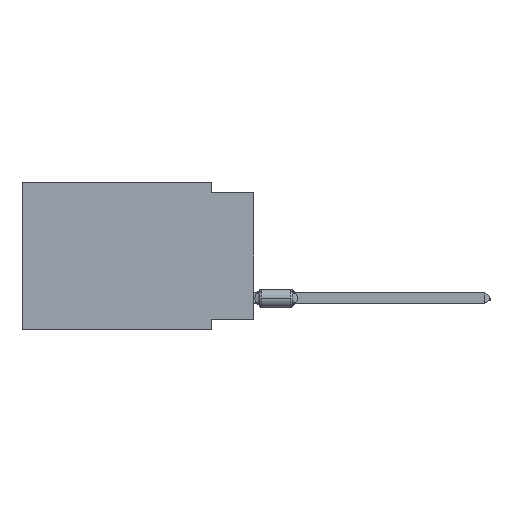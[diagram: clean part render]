
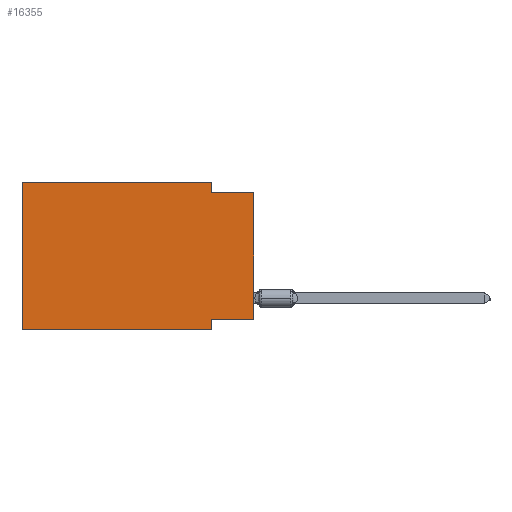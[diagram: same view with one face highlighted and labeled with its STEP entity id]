
A CAD part, left-side view. The second image highlights one B-rep face of the part: STEP entity #16355.
In plain terms, the highlighted planar face has unit normal (-1, 0, 0).
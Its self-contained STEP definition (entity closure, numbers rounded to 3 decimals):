
#432 = CARTESIAN_POINT ( 'NONE',  ( 0., 2.54, 0. ) ) ;
#1191 = EDGE_LOOP ( 'NONE', ( #4856, #4964, #36572, #7061, #2032, #25791, #12695, #21162 ) ) ;
#1422 = VERTEX_POINT ( 'NONE', #13191 ) ;
#2032 = ORIENTED_EDGE ( 'NONE', *, *, #30487, .F. ) ;
#3609 = VERTEX_POINT ( 'NONE', #37012 ) ;
#4856 = ORIENTED_EDGE ( 'NONE', *, *, #19941, .T. ) ;
#4964 = ORIENTED_EDGE ( 'NONE', *, *, #16062, .F. ) ;
#5283 = CARTESIAN_POINT ( 'NONE',  ( 0., 13.97, 0. ) ) ;
#6140 = VECTOR ( 'NONE', #25593, 1000. ) ;
#7061 = ORIENTED_EDGE ( 'NONE', *, *, #39966, .F. ) ;
#8641 = DIRECTION ( 'NONE',  ( 0., 0., -1. ) ) ;
#8751 = DIRECTION ( 'NONE',  ( 1., 0., 0. ) ) ;
#8775 = VERTEX_POINT ( 'NONE', #19262 ) ;
#9508 = DIRECTION ( 'NONE',  ( 0., 0., 1. ) ) ;
#9916 = VERTEX_POINT ( 'NONE', #18288 ) ;
#9973 = LINE ( 'NONE', #16452, #18330 ) ;
#10069 = DIRECTION ( 'NONE',  ( 0., -1., 0. ) ) ;
#10110 = CARTESIAN_POINT ( 'NONE',  ( 0., 0., -8.255 ) ) ;
#11424 = CARTESIAN_POINT ( 'NONE',  ( 0., 0., 0. ) ) ;
#12224 = PLANE ( 'NONE',  #42562 ) ;
#12229 = VERTEX_POINT ( 'NONE', #25708 ) ;
#12476 = CARTESIAN_POINT ( 'NONE',  ( 0., 13.97, 0. ) ) ;
#12695 = ORIENTED_EDGE ( 'NONE', *, *, #37473, .F. ) ;
#13191 = CARTESIAN_POINT ( 'NONE',  ( 0., 2.54, -0.635 ) ) ;
#13728 = EDGE_CURVE ( 'NONE', #8775, #12229, #27521, .T. ) ;
#15688 = VECTOR ( 'NONE', #30538, 1000. ) ;
#16062 = EDGE_CURVE ( 'NONE', #1422, #30753, #19917, .T. ) ;
#16355 = ADVANCED_FACE ( 'NONE', ( #44073 ), #12224, .F. ) ;
#16418 = LINE ( 'NONE', #12476, #29324 ) ;
#16452 = CARTESIAN_POINT ( 'NONE',  ( 0., 13.97, 0. ) ) ;
#16458 = CARTESIAN_POINT ( 'NONE',  ( 0., 0., -0.635 ) ) ;
#16690 = VERTEX_POINT ( 'NONE', #432 ) ;
#17000 = CARTESIAN_POINT ( 'NONE',  ( 0., 13.97, -8.89 ) ) ;
#18288 = CARTESIAN_POINT ( 'NONE',  ( 0., 13.97, -8.89 ) ) ;
#18330 = VECTOR ( 'NONE', #9508, 1000. ) ;
#19262 = CARTESIAN_POINT ( 'NONE',  ( 0., 0., -8.255 ) ) ;
#19917 = LINE ( 'NONE', #16458, #41046 ) ;
#19941 = EDGE_CURVE ( 'NONE', #8775, #30753, #43264, .T. ) ;
#21162 = ORIENTED_EDGE ( 'NONE', *, *, #13728, .F. ) ;
#21910 = VERTEX_POINT ( 'NONE', #25066 ) ;
#22568 = LINE ( 'NONE', #33264, #24740 ) ;
#22686 = EDGE_CURVE ( 'NONE', #16690, #1422, #22568, .T. ) ;
#23997 = LINE ( 'NONE', #17000, #28843 ) ;
#24740 = VECTOR ( 'NONE', #8641, 1000. ) ;
#25066 = CARTESIAN_POINT ( 'NONE',  ( 0., 13.97, 0. ) ) ;
#25593 = DIRECTION ( 'NONE',  ( 0., 0., 1. ) ) ;
#25708 = CARTESIAN_POINT ( 'NONE',  ( 0., 2.54, -8.255 ) ) ;
#25791 = ORIENTED_EDGE ( 'NONE', *, *, #32150, .T. ) ;
#27495 = LINE ( 'NONE', #37737, #15688 ) ;
#27521 = LINE ( 'NONE', #10110, #37944 ) ;
#28843 = VECTOR ( 'NONE', #10069, 1000. ) ;
#29324 = VECTOR ( 'NONE', #44798, 1000. ) ;
#30487 = EDGE_CURVE ( 'NONE', #9916, #21910, #9973, .T. ) ;
#30538 = DIRECTION ( 'NONE',  ( 0., 0., -1. ) ) ;
#30660 = DIRECTION ( 'NONE',  ( 0., -1., 0. ) ) ;
#30753 = VERTEX_POINT ( 'NONE', #32472 ) ;
#32150 = EDGE_CURVE ( 'NONE', #9916, #3609, #23997, .T. ) ;
#32472 = CARTESIAN_POINT ( 'NONE',  ( 0., 0., -0.635 ) ) ;
#33264 = CARTESIAN_POINT ( 'NONE',  ( 0., 2.54, 0. ) ) ;
#36572 = ORIENTED_EDGE ( 'NONE', *, *, #22686, .F. ) ;
#37012 = CARTESIAN_POINT ( 'NONE',  ( 0., 2.54, -8.89 ) ) ;
#37473 = EDGE_CURVE ( 'NONE', #12229, #3609, #27495, .T. ) ;
#37737 = CARTESIAN_POINT ( 'NONE',  ( 0., 2.54, -8.89 ) ) ;
#37944 = VECTOR ( 'NONE', #45418, 1000. ) ;
#39966 = EDGE_CURVE ( 'NONE', #21910, #16690, #16418, .T. ) ;
#40582 = DIRECTION ( 'NONE',  ( 0., 0., -1. ) ) ;
#41046 = VECTOR ( 'NONE', #30660, 1000. ) ;
#42562 = AXIS2_PLACEMENT_3D ( 'NONE', #5283, #8751, #40582 ) ;
#43264 = LINE ( 'NONE', #11424, #6140 ) ;
#44073 = FACE_OUTER_BOUND ( 'NONE', #1191, .T. ) ;
#44798 = DIRECTION ( 'NONE',  ( 0., -1., 0. ) ) ;
#45418 = DIRECTION ( 'NONE',  ( 0., 1., 0. ) ) ;
